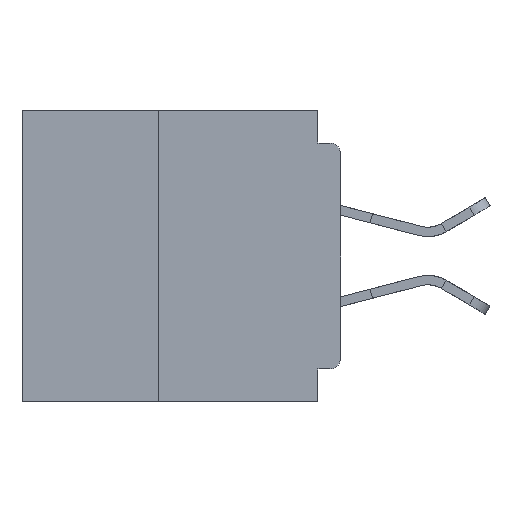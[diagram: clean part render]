
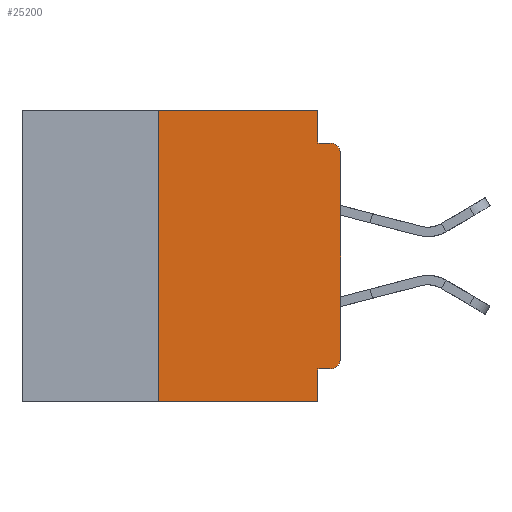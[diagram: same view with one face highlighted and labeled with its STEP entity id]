
A CAD part, left-side view. The second image highlights one B-rep face of the part: STEP entity #25200.
In plain terms, the highlighted planar face has unit normal (-1, 0, 0).
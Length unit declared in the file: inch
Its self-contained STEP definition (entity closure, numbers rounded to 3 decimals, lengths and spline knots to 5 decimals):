
#145 = VERTEX_POINT ( 'NONE', #15003 ) ;
#191 = CARTESIAN_POINT ( 'NONE',  ( 0., 0.015, -0.34 ) ) ;
#205 = EDGE_CURVE ( 'NONE', #28730, #145, #25323, .T. ) ;
#303 = ORIENTED_EDGE ( 'NONE', *, *, #18544, .F. ) ;
#652 = AXIS2_PLACEMENT_3D ( 'NONE', #21888, #2993, #25025 ) ;
#699 = VERTEX_POINT ( 'NONE', #36439 ) ;
#1627 = EDGE_CURVE ( 'NONE', #22627, #8085, #18330, .T. ) ;
#1969 = CARTESIAN_POINT ( 'NONE',  ( 0., 0., -0.355 ) ) ;
#2359 = DIRECTION ( 'NONE',  ( 0., 0., -1. ) ) ;
#2993 = DIRECTION ( 'NONE',  ( -1., 0., 0. ) ) ;
#3386 = DIRECTION ( 'NONE',  ( 0., 0., -1. ) ) ;
#3764 = ORIENTED_EDGE ( 'NONE', *, *, #9567, .F. ) ;
#4330 = CARTESIAN_POINT ( 'NONE',  ( 0., 0., -0.06 ) ) ;
#5039 = DIRECTION ( 'NONE',  ( 0., 0., -1. ) ) ;
#6214 = LINE ( 'NONE', #31072, #39477 ) ;
#7114 = VERTEX_POINT ( 'NONE', #8666 ) ;
#7164 = ORIENTED_EDGE ( 'NONE', *, *, #8488, .T. ) ;
#8085 = VERTEX_POINT ( 'NONE', #4330 ) ;
#8269 = DIRECTION ( 'NONE',  ( 0., 1., 0. ) ) ;
#8488 = EDGE_CURVE ( 'NONE', #8085, #7114, #34574, .T. ) ;
#8666 = CARTESIAN_POINT ( 'NONE',  ( 0., 0.015, -0.045 ) ) ;
#8693 = ORIENTED_EDGE ( 'NONE', *, *, #27983, .T. ) ;
#9378 = EDGE_CURVE ( 'NONE', #10042, #145, #36416, .T. ) ;
#9567 = EDGE_CURVE ( 'NONE', #36210, #33559, #28665, .T. ) ;
#9892 = VECTOR ( 'NONE', #35759, 39.37008 ) ;
#10042 = VERTEX_POINT ( 'NONE', #10991 ) ;
#10407 = EDGE_CURVE ( 'NONE', #33559, #19746, #20327, .T. ) ;
#10991 = CARTESIAN_POINT ( 'NONE',  ( 0., 0.25, -0.4 ) ) ;
#12152 = ORIENTED_EDGE ( 'NONE', *, *, #21504, .F. ) ;
#12306 = AXIS2_PLACEMENT_3D ( 'NONE', #18073, #21236, #2359 ) ;
#14128 = ORIENTED_EDGE ( 'NONE', *, *, #9378, .T. ) ;
#14888 = PLANE ( 'NONE',  #12306 ) ;
#15003 = CARTESIAN_POINT ( 'NONE',  ( 0., 0.031, -0.4 ) ) ;
#15332 = CARTESIAN_POINT ( 'NONE',  ( 0., 0.031, -0.4 ) ) ;
#17422 = DIRECTION ( 'NONE',  ( 0., -1., 0. ) ) ;
#17604 = ORIENTED_EDGE ( 'NONE', *, *, #27925, .F. ) ;
#18073 = CARTESIAN_POINT ( 'NONE',  ( 0., 0.437, 0. ) ) ;
#18330 = LINE ( 'NONE', #25921, #9892 ) ;
#18544 = EDGE_CURVE ( 'NONE', #699, #28730, #36529, .T. ) ;
#18942 = VECTOR ( 'NONE', #17422, 39.37008 ) ;
#18985 = CARTESIAN_POINT ( 'NONE',  ( 0., 0.031, 0. ) ) ;
#19043 = VECTOR ( 'NONE', #8269, 39.37008 ) ;
#19283 = CARTESIAN_POINT ( 'NONE',  ( 0., 0., -0.34 ) ) ;
#19363 = CARTESIAN_POINT ( 'NONE',  ( 0., 0.25, 0. ) ) ;
#19746 = VERTEX_POINT ( 'NONE', #21044 ) ;
#20327 = LINE ( 'NONE', #18985, #26670 ) ;
#21044 = CARTESIAN_POINT ( 'NONE',  ( 0., 0.031, -0.045 ) ) ;
#21236 = DIRECTION ( 'NONE',  ( 1., 0., 0. ) ) ;
#21414 = VECTOR ( 'NONE', #5039, 39.37008 ) ;
#21504 = EDGE_CURVE ( 'NONE', #10042, #36210, #39186, .T. ) ;
#21881 = DIRECTION ( 'NONE',  ( 0., -1., 0. ) ) ;
#21888 = CARTESIAN_POINT ( 'NONE',  ( 0., 0.015, -0.06 ) ) ;
#22253 = DIRECTION ( 'NONE',  ( -1., 0., 0. ) ) ;
#22493 = ORIENTED_EDGE ( 'NONE', *, *, #205, .F. ) ;
#22627 = VERTEX_POINT ( 'NONE', #19283 ) ;
#22711 = VECTOR ( 'NONE', #29600, 39.37008 ) ;
#23246 = FACE_OUTER_BOUND ( 'NONE', #36847, .T. ) ;
#24549 = CARTESIAN_POINT ( 'NONE',  ( 0., 0.437, 0. ) ) ;
#25025 = DIRECTION ( 'NONE',  ( 0., 0., -1. ) ) ;
#25200 = ADVANCED_FACE ( 'NONE', ( #23246 ), #14888, .F. ) ;
#25323 = LINE ( 'NONE', #15332, #21414 ) ;
#25921 = CARTESIAN_POINT ( 'NONE',  ( 0., 0., 0. ) ) ;
#26490 = CARTESIAN_POINT ( 'NONE',  ( 0., 0.25, -0.4 ) ) ;
#26670 = VECTOR ( 'NONE', #31486, 39.37008 ) ;
#27654 = DIRECTION ( 'NONE',  ( 0., -1., 0. ) ) ;
#27724 = VECTOR ( 'NONE', #27654, 39.37008 ) ;
#27925 = EDGE_CURVE ( 'NONE', #19746, #7114, #6214, .T. ) ;
#27983 = EDGE_CURVE ( 'NONE', #699, #22627, #35556, .T. ) ;
#28665 = LINE ( 'NONE', #24549, #27724 ) ;
#28730 = VERTEX_POINT ( 'NONE', #32373 ) ;
#29600 = DIRECTION ( 'NONE',  ( 0., 0., 1. ) ) ;
#30792 = AXIS2_PLACEMENT_3D ( 'NONE', #191, #22253, #3386 ) ;
#31072 = CARTESIAN_POINT ( 'NONE',  ( 0., 0., -0.045 ) ) ;
#31486 = DIRECTION ( 'NONE',  ( 0., 0., -1. ) ) ;
#32373 = CARTESIAN_POINT ( 'NONE',  ( 0., 0.031, -0.355 ) ) ;
#32918 = CARTESIAN_POINT ( 'NONE',  ( 0., 0.437, -0.4 ) ) ;
#33559 = VERTEX_POINT ( 'NONE', #38431 ) ;
#34140 = ORIENTED_EDGE ( 'NONE', *, *, #10407, .F. ) ;
#34574 = CIRCLE ( 'NONE', #652, 0.015 ) ;
#35556 = CIRCLE ( 'NONE', #30792, 0.015 ) ;
#35759 = DIRECTION ( 'NONE',  ( 0., 0., 1. ) ) ;
#36210 = VERTEX_POINT ( 'NONE', #19363 ) ;
#36416 = LINE ( 'NONE', #32918, #18942 ) ;
#36439 = CARTESIAN_POINT ( 'NONE',  ( 0., 0.015, -0.355 ) ) ;
#36529 = LINE ( 'NONE', #1969, #19043 ) ;
#36847 = EDGE_LOOP ( 'NONE', ( #39448, #7164, #17604, #34140, #3764, #12152, #14128, #22493, #303, #8693 ) ) ;
#38431 = CARTESIAN_POINT ( 'NONE',  ( 0., 0.031, 0. ) ) ;
#39186 = LINE ( 'NONE', #26490, #22711 ) ;
#39448 = ORIENTED_EDGE ( 'NONE', *, *, #1627, .T. ) ;
#39477 = VECTOR ( 'NONE', #21881, 39.37008 ) ;
